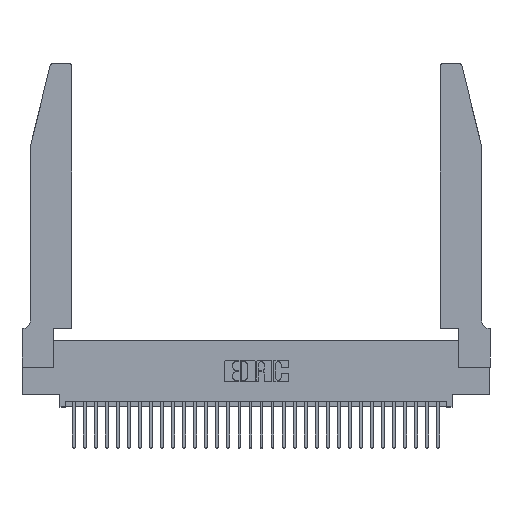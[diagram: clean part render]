
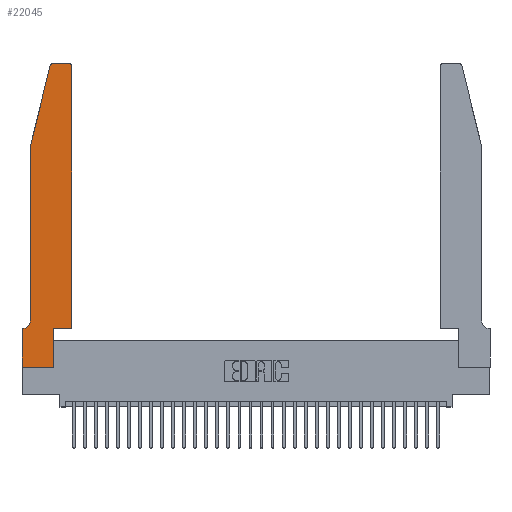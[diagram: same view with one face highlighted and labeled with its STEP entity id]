
A CAD part, top view. The second image highlights one B-rep face of the part: STEP entity #22045.
In plain terms, the highlighted planar face has unit normal (0, 0, 1).
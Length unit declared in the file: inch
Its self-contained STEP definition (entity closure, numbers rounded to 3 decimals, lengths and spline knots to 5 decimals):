
#194 = EDGE_CURVE ( 'NONE', #20299, #21765, #19703, .T. ) ;
#313 = CARTESIAN_POINT ( 'NONE',  ( 0.2865, 0.35, 0.37 ) ) ;
#633 = AXIS2_PLACEMENT_3D ( 'NONE', #22898, #30343, #25245 ) ;
#872 = ORIENTED_EDGE ( 'NONE', *, *, #16618, .T. ) ;
#1415 = ORIENTED_EDGE ( 'NONE', *, *, #16158, .T. ) ;
#2742 = CARTESIAN_POINT ( 'NONE',  ( 0.4505, 0.35, 0.37 ) ) ;
#3001 = LINE ( 'NONE', #4135, #20428 ) ;
#3136 = CARTESIAN_POINT ( 'NONE',  ( 0.4205, 2.75, 0.37 ) ) ;
#3155 = EDGE_CURVE ( 'NONE', #20537, #15332, #3259, .T. ) ;
#3259 = LINE ( 'NONE', #25182, #8817 ) ;
#3650 = CARTESIAN_POINT ( 'NONE',  ( 0., 0.35, 0.37 ) ) ;
#4054 = LINE ( 'NONE', #2742, #26987 ) ;
#4081 = VECTOR ( 'NONE', #23036, 39.37008 ) ;
#4135 = CARTESIAN_POINT ( 'NONE',  ( 0.2605, 2.75, 0.37 ) ) ;
#4146 = DIRECTION ( 'NONE',  ( 0., 1., 0. ) ) ;
#4721 = FACE_OUTER_BOUND ( 'NONE', #27293, .T. ) ;
#5071 = PLANE ( 'NONE',  #28199 ) ;
#5609 = DIRECTION ( 'NONE',  ( -0.239, -0.971, 0. ) ) ;
#6026 = LINE ( 'NONE', #313, #4081 ) ;
#6540 = ORIENTED_EDGE ( 'NONE', *, *, #26415, .T. ) ;
#6589 = DIRECTION ( 'NONE',  ( 1., 0., 0. ) ) ;
#7074 = CARTESIAN_POINT ( 'NONE',  ( 0.0755, 0.35, 0.37 ) ) ;
#7532 = EDGE_CURVE ( 'NONE', #26455, #31561, #14480, .T. ) ;
#7620 = DIRECTION ( 'NONE',  ( 1., 0., 0. ) ) ;
#7673 = ORIENTED_EDGE ( 'NONE', *, *, #3155, .T. ) ;
#8079 = VERTEX_POINT ( 'NONE', #21476 ) ;
#8396 = ORIENTED_EDGE ( 'NONE', *, *, #20137, .T. ) ;
#8817 = VECTOR ( 'NONE', #7620, 39.37008 ) ;
#9259 = ORIENTED_EDGE ( 'NONE', *, *, #18439, .T. ) ;
#9319 = CARTESIAN_POINT ( 'NONE',  ( 0.0055, 0.35, 0.37 ) ) ;
#10287 = VERTEX_POINT ( 'NONE', #19382 ) ;
#10952 = LINE ( 'NONE', #22999, #13281 ) ;
#11622 = CIRCLE ( 'NONE', #633, 0.03 ) ;
#12199 = CARTESIAN_POINT ( 'NONE',  ( 0.4505, 2.72, 0.37 ) ) ;
#12736 = LINE ( 'NONE', #25692, #28553 ) ;
#13281 = VECTOR ( 'NONE', #25335, 39.37008 ) ;
#13411 = EDGE_CURVE ( 'NONE', #31561, #20537, #25125, .T. ) ;
#14393 = CARTESIAN_POINT ( 'NONE',  ( 0.0755, 0.42, 0.37 ) ) ;
#14480 = LINE ( 'NONE', #7074, #28299 ) ;
#14643 = DIRECTION ( 'NONE',  ( -1., 0., 0. ) ) ;
#15043 = LINE ( 'NONE', #24114, #20204 ) ;
#15332 = VERTEX_POINT ( 'NONE', #18600 ) ;
#15554 = CARTESIAN_POINT ( 'NONE',  ( 0.0755, 2., 0.37 ) ) ;
#15607 = VECTOR ( 'NONE', #23195, 39.37008 ) ;
#16144 = EDGE_CURVE ( 'NONE', #31554, #24467, #12736, .T. ) ;
#16158 = EDGE_CURVE ( 'NONE', #15332, #10287, #6026, .T. ) ;
#16618 = EDGE_CURVE ( 'NONE', #24467, #29610, #10952, .T. ) ;
#17140 = DIRECTION ( 'NONE',  ( -1., 0., 0. ) ) ;
#18439 = EDGE_CURVE ( 'NONE', #25432, #31554, #11622, .T. ) ;
#18600 = CARTESIAN_POINT ( 'NONE',  ( 0.2865, 0., 0.37 ) ) ;
#18906 = ORIENTED_EDGE ( 'NONE', *, *, #16144, .T. ) ;
#18989 = CARTESIAN_POINT ( 'NONE',  ( 0.25487, 2.72718, 0.37 ) ) ;
#19143 = DIRECTION ( 'NONE',  ( -1., 0., 0. ) ) ;
#19382 = CARTESIAN_POINT ( 'NONE',  ( 0.2865, 0.35, 0.37 ) ) ;
#19703 = CIRCLE ( 'NONE', #32446, 0.03 ) ;
#19853 = DIRECTION ( 'NONE',  ( 1., 0., 0. ) ) ;
#20093 = CARTESIAN_POINT ( 'NONE',  ( 0.284, 2.75, 0.37 ) ) ;
#20137 = EDGE_CURVE ( 'NONE', #29610, #26455, #20206, .T. ) ;
#20178 = CARTESIAN_POINT ( 'NONE',  ( 0., 0.35, 0.37 ) ) ;
#20204 = VECTOR ( 'NONE', #4146, 39.37008 ) ;
#20206 = CIRCLE ( 'NONE', #27099, 0.07 ) ;
#20262 = DIRECTION ( 'NONE',  ( 0., 0., 1. ) ) ;
#20299 = VERTEX_POINT ( 'NONE', #12199 ) ;
#20428 = VECTOR ( 'NONE', #19143, 39.37008 ) ;
#20537 = VERTEX_POINT ( 'NONE', #28498 ) ;
#20646 = DIRECTION ( 'NONE',  ( 1., 0., 0. ) ) ;
#20679 = ORIENTED_EDGE ( 'NONE', *, *, #30436, .T. ) ;
#21476 = CARTESIAN_POINT ( 'NONE',  ( 0.4505, 0.35, 0.37 ) ) ;
#21765 = VERTEX_POINT ( 'NONE', #3136 ) ;
#21805 = DIRECTION ( 'NONE',  ( 0., 0., -1. ) ) ;
#22012 = ORIENTED_EDGE ( 'NONE', *, *, #7532, .T. ) ;
#22045 = ADVANCED_FACE ( 'NONE', ( #4721 ), #5071, .T. ) ;
#22898 = CARTESIAN_POINT ( 'NONE',  ( 0.284, 2.72, 0.37 ) ) ;
#22999 = CARTESIAN_POINT ( 'NONE',  ( 0.0755, 2., 0.37 ) ) ;
#23036 = DIRECTION ( 'NONE',  ( 0., 1., 0. ) ) ;
#23195 = DIRECTION ( 'NONE',  ( 0., -1., 0. ) ) ;
#23236 = ORIENTED_EDGE ( 'NONE', *, *, #31183, .T. ) ;
#24114 = CARTESIAN_POINT ( 'NONE',  ( 0.4505, 0.35, 0.37 ) ) ;
#24467 = VERTEX_POINT ( 'NONE', #15554 ) ;
#24558 = CARTESIAN_POINT ( 'NONE',  ( 0.0055, 0.42, 0.37 ) ) ;
#25125 = LINE ( 'NONE', #31613, #15607 ) ;
#25182 = CARTESIAN_POINT ( 'NONE',  ( 0., 0., 0.37 ) ) ;
#25198 = ORIENTED_EDGE ( 'NONE', *, *, #194, .T. ) ;
#25245 = DIRECTION ( 'NONE',  ( 1., 0., 0. ) ) ;
#25335 = DIRECTION ( 'NONE',  ( 0., -1., 0. ) ) ;
#25432 = VERTEX_POINT ( 'NONE', #20093 ) ;
#25692 = CARTESIAN_POINT ( 'NONE',  ( 0.0755, 2., 0.37 ) ) ;
#25754 = CARTESIAN_POINT ( 'NONE',  ( 0.4205, 2.72, 0.37 ) ) ;
#26415 = EDGE_CURVE ( 'NONE', #21765, #25432, #3001, .T. ) ;
#26455 = VERTEX_POINT ( 'NONE', #9319 ) ;
#26987 = VECTOR ( 'NONE', #20646, 39.37008 ) ;
#27099 = AXIS2_PLACEMENT_3D ( 'NONE', #24558, #21805, #17140 ) ;
#27293 = EDGE_LOOP ( 'NONE', ( #6540, #9259, #18906, #872, #8396, #22012, #31441, #7673, #1415, #20679, #23236, #25198 ) ) ;
#28199 = AXIS2_PLACEMENT_3D ( 'NONE', #20178, #30133, #19853 ) ;
#28299 = VECTOR ( 'NONE', #14643, 39.37008 ) ;
#28498 = CARTESIAN_POINT ( 'NONE',  ( 0., 0., 0.37 ) ) ;
#28553 = VECTOR ( 'NONE', #5609, 39.37008 ) ;
#29610 = VERTEX_POINT ( 'NONE', #14393 ) ;
#30133 = DIRECTION ( 'NONE',  ( 0., 0., 1. ) ) ;
#30343 = DIRECTION ( 'NONE',  ( 0., 0., 1. ) ) ;
#30436 = EDGE_CURVE ( 'NONE', #10287, #8079, #4054, .T. ) ;
#31183 = EDGE_CURVE ( 'NONE', #8079, #20299, #15043, .T. ) ;
#31441 = ORIENTED_EDGE ( 'NONE', *, *, #13411, .T. ) ;
#31554 = VERTEX_POINT ( 'NONE', #18989 ) ;
#31561 = VERTEX_POINT ( 'NONE', #3650 ) ;
#31613 = CARTESIAN_POINT ( 'NONE',  ( 0., 0., 0.37 ) ) ;
#32446 = AXIS2_PLACEMENT_3D ( 'NONE', #25754, #20262, #6589 ) ;
